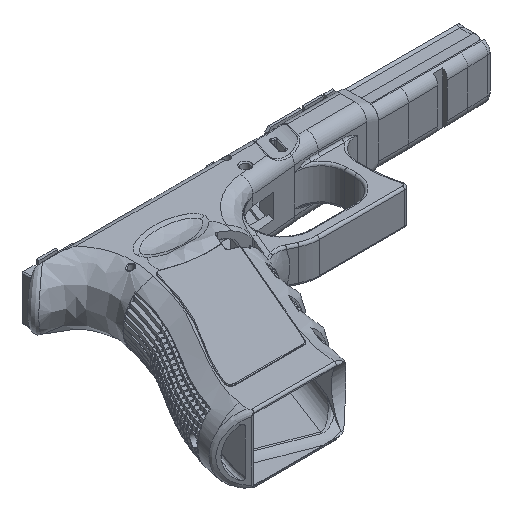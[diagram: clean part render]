
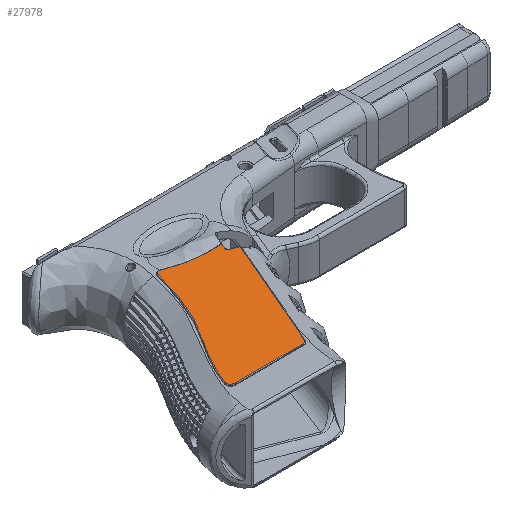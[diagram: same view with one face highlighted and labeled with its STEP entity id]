
A CAD part, isometric view. The second image highlights one B-rep face of the part: STEP entity #27978.
In plain terms, the highlighted planar face has unit normal (0, 0, 1).
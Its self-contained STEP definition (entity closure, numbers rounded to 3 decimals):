
#61=PLANE('',#29914);
#1280=CIRCLE('',#29788,1.27);
#1359=CIRCLE('',#29915,44.824);
#1360=CIRCLE('',#29916,1.778);
#1361=CIRCLE('',#29917,102.555);
#1362=CIRCLE('',#29918,86.316);
#1363=CIRCLE('',#29919,1.778);
#1364=CIRCLE('',#29920,1.778);
#2021=FACE_OUTER_BOUND('',#3871,.T.);
#3871=EDGE_LOOP('',(#19098,#19099,#19100,#19101,#19102,#19103,#19104,#19105,
#19106,#19107,#19108));
#5777=LINE('',#44560,#7844);
#5778=LINE('',#44561,#7845);
#5779=LINE('',#44562,#7846);
#5780=LINE('',#44574,#7847);
#7844=VECTOR('',#31992,1000.);
#7845=VECTOR('',#31993,1000.);
#7846=VECTOR('',#31994,1000.);
#7847=VECTOR('',#32005,1000.);
#11655=VERTEX_POINT('',#38943);
#11658=VERTEX_POINT('',#38950);
#11659=VERTEX_POINT('',#38952);
#11662=VERTEX_POINT('',#38959);
#11943=VERTEX_POINT('',#44559);
#11944=VERTEX_POINT('',#44563);
#11945=VERTEX_POINT('',#44565);
#11946=VERTEX_POINT('',#44567);
#11947=VERTEX_POINT('',#44569);
#11948=VERTEX_POINT('',#44571);
#11949=VERTEX_POINT('',#44573);
#14237=EDGE_CURVE('',#11659,#11658,#1280,.T.);
#14581=EDGE_CURVE('',#11662,#11943,#5777,.T.);
#14582=EDGE_CURVE('',#11662,#11659,#5778,.T.);
#14583=EDGE_CURVE('',#11658,#11655,#5779,.T.);
#14584=EDGE_CURVE('',#11944,#11655,#1359,.T.);
#14585=EDGE_CURVE('',#11945,#11944,#1360,.T.);
#14586=EDGE_CURVE('',#11946,#11945,#1361,.T.);
#14587=EDGE_CURVE('',#11947,#11946,#1362,.T.);
#14588=EDGE_CURVE('',#11948,#11947,#1363,.T.);
#14589=EDGE_CURVE('',#11949,#11948,#5780,.T.);
#14590=EDGE_CURVE('',#11943,#11949,#1364,.T.);
#19098=ORIENTED_EDGE('',*,*,#14581,.F.);
#19099=ORIENTED_EDGE('',*,*,#14582,.T.);
#19100=ORIENTED_EDGE('',*,*,#14237,.T.);
#19101=ORIENTED_EDGE('',*,*,#14583,.T.);
#19102=ORIENTED_EDGE('',*,*,#14584,.F.);
#19103=ORIENTED_EDGE('',*,*,#14585,.F.);
#19104=ORIENTED_EDGE('',*,*,#14586,.F.);
#19105=ORIENTED_EDGE('',*,*,#14587,.F.);
#19106=ORIENTED_EDGE('',*,*,#14588,.F.);
#19107=ORIENTED_EDGE('',*,*,#14589,.F.);
#19108=ORIENTED_EDGE('',*,*,#14590,.F.);
#27978=ADVANCED_FACE('',(#2021),#61,.F.);
#29788=AXIS2_PLACEMENT_3D('',#38953,#31638,#31639);
#29914=AXIS2_PLACEMENT_3D('',#44558,#31990,#31991);
#29915=AXIS2_PLACEMENT_3D('',#44564,#31995,#31996);
#29916=AXIS2_PLACEMENT_3D('',#44566,#31997,#31998);
#29917=AXIS2_PLACEMENT_3D('',#44568,#31999,#32000);
#29918=AXIS2_PLACEMENT_3D('',#44570,#32001,#32002);
#29919=AXIS2_PLACEMENT_3D('',#44572,#32003,#32004);
#29920=AXIS2_PLACEMENT_3D('',#44575,#32006,#32007);
#31638=DIRECTION('center_axis',(0.,0.,
-1.));
#31639=DIRECTION('ref_axis',(-1.,0.,0.));
#31990=DIRECTION('center_axis',(0.,0.,
-1.));
#31991=DIRECTION('ref_axis',(1.,0.,0.));
#31992=DIRECTION('',(-0.396,-0.918,0.));
#31993=DIRECTION('',(-0.934,0.358,0.));
#31994=DIRECTION('',(0.358,0.934,0.));
#31995=DIRECTION('center_axis',(0.,0.,
1.));
#31996=DIRECTION('ref_axis',(1.,0.,0.));
#31997=DIRECTION('center_axis',(0.,0.,
-1.));
#31998=DIRECTION('ref_axis',(1.,0.,0.));
#31999=DIRECTION('center_axis',(0.,0.,
1.));
#32000=DIRECTION('ref_axis',(1.,0.,0.));
#32001=DIRECTION('center_axis',(0.,0.,
-1.));
#32002=DIRECTION('ref_axis',(1.,0.,0.));
#32003=DIRECTION('center_axis',(0.,0.,
-1.));
#32004=DIRECTION('ref_axis',(1.,0.,0.));
#32005=DIRECTION('',(-1.,0.,0.));
#32006=DIRECTION('center_axis',(0.,0.,
-1.));
#32007=DIRECTION('ref_axis',(1.,0.,0.));
#38943=CARTESIAN_POINT('',(54.494,67.354,14.941));
#38950=CARTESIAN_POINT('',(53.68,65.234,14.941));
#38952=CARTESIAN_POINT('',(54.41,63.593,14.941));
#38953=CARTESIAN_POINT('Origin',(54.865,64.779,14.941));
#38959=CARTESIAN_POINT('',(57.5,62.407,14.941));
#44558=CARTESIAN_POINT('Origin',(85.161,-14.94,14.941));
#44559=CARTESIAN_POINT('',(36.884,14.537,14.941));
#44560=CARTESIAN_POINT('',(36.884,14.537,14.941));
#44561=CARTESIAN_POINT('',(54.41,63.593,14.941));
#44562=CARTESIAN_POINT('',(54.541,67.477,14.941));
#44563=CARTESIAN_POINT('',(32.235,70.631,14.941));
#44564=CARTESIAN_POINT('Origin',(49.685,111.919,14.941));
#44565=CARTESIAN_POINT('',(29.811,69.397,14.941));
#44566=CARTESIAN_POINT('Origin',(31.543,68.994,14.941));
#44567=CARTESIAN_POINT('',(14.217,34.226,14.941));
#44568=CARTESIAN_POINT('Origin',(-70.075,92.642,14.941));
#44569=CARTESIAN_POINT('',(4.534,15.875,14.941));
#44570=CARTESIAN_POINT('Origin',(85.161,-14.94,14.941));
#44571=CARTESIAN_POINT('',(6.194,13.462,14.941));
#44572=CARTESIAN_POINT('Origin',(6.194,15.24,14.941));
#44573=CARTESIAN_POINT('',(35.251,13.462,14.941));
#44574=CARTESIAN_POINT('',(6.194,13.462,14.941));
#44575=CARTESIAN_POINT('Origin',(35.251,15.24,14.941));
